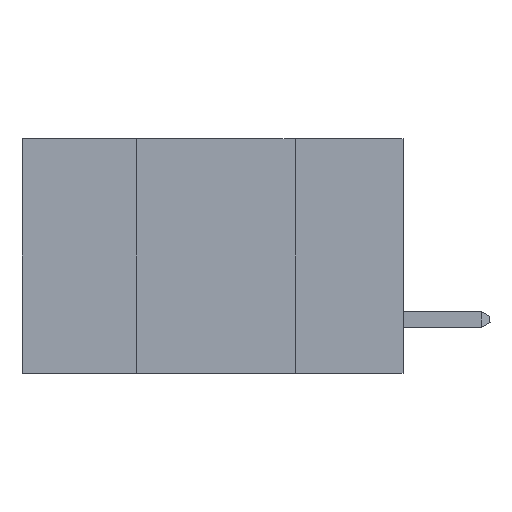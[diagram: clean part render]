
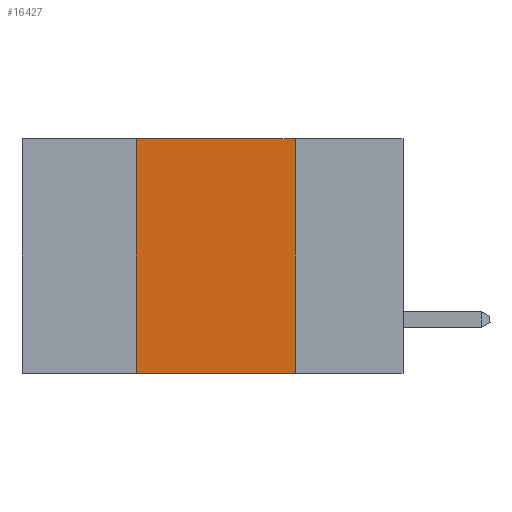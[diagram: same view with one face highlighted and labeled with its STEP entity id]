
A CAD part, left-side view. The second image highlights one B-rep face of the part: STEP entity #16427.
In plain terms, the highlighted planar face has unit normal (-1, 0, 0).
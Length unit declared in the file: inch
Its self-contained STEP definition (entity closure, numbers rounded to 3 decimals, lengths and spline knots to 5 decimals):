
#1574 = ORIENTED_EDGE ( 'NONE', *, *, #20295, .F. ) ;
#2374 = VERTEX_POINT ( 'NONE', #25232 ) ;
#4012 = EDGE_CURVE ( 'NONE', #4664, #4770, #13498, .T. ) ;
#4210 = CARTESIAN_POINT ( 'NONE',  ( 0., 0.6, 0. ) ) ;
#4664 = VERTEX_POINT ( 'NONE', #25148 ) ;
#4684 = CARTESIAN_POINT ( 'NONE',  ( 0., 0.6, 0. ) ) ;
#4770 = VERTEX_POINT ( 'NONE', #12929 ) ;
#5891 = VECTOR ( 'NONE', #16567, 39.37008 ) ;
#6178 = PLANE ( 'NONE',  #22415 ) ;
#6262 = DIRECTION ( 'NONE',  ( 0., 0., -1. ) ) ;
#7286 = CARTESIAN_POINT ( 'NONE',  ( 0., 0.6, -0.37 ) ) ;
#7861 = LINE ( 'NONE', #7286, #18280 ) ;
#8204 = CARTESIAN_POINT ( 'NONE',  ( 0., 0.17, 0. ) ) ;
#9566 = VECTOR ( 'NONE', #13526, 39.37008 ) ;
#10009 = EDGE_LOOP ( 'NONE', ( #22560, #21983, #1574, #22272 ) ) ;
#10199 = FACE_OUTER_BOUND ( 'NONE', #10009, .T. ) ;
#11728 = LINE ( 'NONE', #4684, #5891 ) ;
#12929 = CARTESIAN_POINT ( 'NONE',  ( 0., 0.17, -0.37 ) ) ;
#13498 = LINE ( 'NONE', #8204, #23189 ) ;
#13526 = DIRECTION ( 'NONE',  ( 0., 0., 1. ) ) ;
#15310 = CARTESIAN_POINT ( 'NONE',  ( 0., 0.42, -0.37 ) ) ;
#15484 = VERTEX_POINT ( 'NONE', #15310 ) ;
#15526 = CARTESIAN_POINT ( 'NONE',  ( 0., 0.42, 0. ) ) ;
#16427 = ADVANCED_FACE ( 'NONE', ( #10199 ), #6178, .F. ) ;
#16567 = DIRECTION ( 'NONE',  ( 0., -1., 0. ) ) ;
#18040 = DIRECTION ( 'NONE',  ( 1., 0., 0. ) ) ;
#18280 = VECTOR ( 'NONE', #20911, 39.37008 ) ;
#19952 = LINE ( 'NONE', #15526, #9566 ) ;
#20009 = EDGE_CURVE ( 'NONE', #2374, #4664, #11728, .T. ) ;
#20295 = EDGE_CURVE ( 'NONE', #15484, #2374, #19952, .T. ) ;
#20659 = DIRECTION ( 'NONE',  ( 0., 0., -1. ) ) ;
#20911 = DIRECTION ( 'NONE',  ( 0., -1., 0. ) ) ;
#21983 = ORIENTED_EDGE ( 'NONE', *, *, #20009, .F. ) ;
#22272 = ORIENTED_EDGE ( 'NONE', *, *, #25512, .T. ) ;
#22415 = AXIS2_PLACEMENT_3D ( 'NONE', #4210, #18040, #6262 ) ;
#22560 = ORIENTED_EDGE ( 'NONE', *, *, #4012, .F. ) ;
#23189 = VECTOR ( 'NONE', #20659, 39.37008 ) ;
#25148 = CARTESIAN_POINT ( 'NONE',  ( 0., 0.17, 0. ) ) ;
#25232 = CARTESIAN_POINT ( 'NONE',  ( 0., 0.42, 0. ) ) ;
#25512 = EDGE_CURVE ( 'NONE', #15484, #4770, #7861, .T. ) ;
